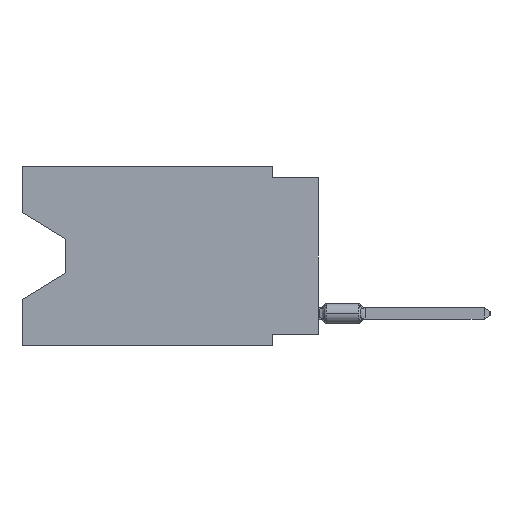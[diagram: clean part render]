
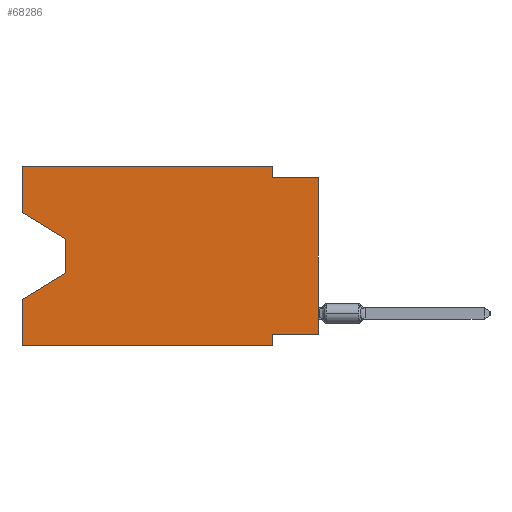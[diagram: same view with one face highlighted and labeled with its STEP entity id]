
A CAD part, left-side view. The second image highlights one B-rep face of the part: STEP entity #68286.
In plain terms, the highlighted planar face has unit normal (-1, 0, 0).
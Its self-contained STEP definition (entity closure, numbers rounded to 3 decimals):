
#536 = DIRECTION ( 'NONE',  ( 0., 0., -1. ) ) ;
#2184 = VECTOR ( 'NONE', #11105, 1000. ) ;
#2478 = EDGE_LOOP ( 'NONE', ( #61921, #39847, #47385, #11487, #75316, #33897, #19832, #38276, #31860, #69973, #53707, #51297 ) ) ;
#2851 = CARTESIAN_POINT ( 'NONE',  ( 0., 13.97, -4.013 ) ) ;
#3075 = EDGE_CURVE ( 'NONE', #68480, #20367, #23605, .T. ) ;
#3220 = VECTOR ( 'NONE', #50101, 1000. ) ;
#3346 = CARTESIAN_POINT ( 'NONE',  ( 0., 16.383, -9.906 ) ) ;
#4246 = DIRECTION ( 'NONE',  ( 0., -0.855, -0.519 ) ) ;
#6321 = CARTESIAN_POINT ( 'NONE',  ( 0., 16.383, 0. ) ) ;
#6379 = VECTOR ( 'NONE', #55084, 1000. ) ;
#6988 = EDGE_CURVE ( 'NONE', #44244, #68480, #17265, .T. ) ;
#7427 = VERTEX_POINT ( 'NONE', #64500 ) ;
#8883 = VERTEX_POINT ( 'NONE', #2851 ) ;
#10782 = CARTESIAN_POINT ( 'NONE',  ( 0., 2.54, -9.271 ) ) ;
#11105 = DIRECTION ( 'NONE',  ( 0., 1., 0. ) ) ;
#11487 = ORIENTED_EDGE ( 'NONE', *, *, #60969, .F. ) ;
#12878 = CARTESIAN_POINT ( 'NONE',  ( 0., 13.97, -4.013 ) ) ;
#13139 = LINE ( 'NONE', #38212, #6379 ) ;
#14327 = VERTEX_POINT ( 'NONE', #59065 ) ;
#14853 = LINE ( 'NONE', #53460, #24360 ) ;
#17265 = LINE ( 'NONE', #54662, #2184 ) ;
#17700 = EDGE_CURVE ( 'NONE', #64147, #47741, #14853, .T. ) ;
#17782 = CARTESIAN_POINT ( 'NONE',  ( 0., 16.383, -7.36 ) ) ;
#19370 = AXIS2_PLACEMENT_3D ( 'NONE', #6321, #31409, #25217 ) ;
#19832 = ORIENTED_EDGE ( 'NONE', *, *, #6988, .F. ) ;
#20367 = VERTEX_POINT ( 'NONE', #27792 ) ;
#20667 = DIRECTION ( 'NONE',  ( 0., 0., 1. ) ) ;
#22752 = DIRECTION ( 'NONE',  ( 0., -1., 0. ) ) ;
#23605 = LINE ( 'NONE', #79504, #75189 ) ;
#24106 = VERTEX_POINT ( 'NONE', #53067 ) ;
#24360 = VECTOR ( 'NONE', #71164, 1000. ) ;
#24638 = CARTESIAN_POINT ( 'NONE',  ( 0., 13.97, -5.893 ) ) ;
#25217 = DIRECTION ( 'NONE',  ( 0., 0., -1. ) ) ;
#26375 = CARTESIAN_POINT ( 'NONE',  ( 0., 0., 0. ) ) ;
#27792 = CARTESIAN_POINT ( 'NONE',  ( 0., 2.54, -9.906 ) ) ;
#28436 = CARTESIAN_POINT ( 'NONE',  ( 0., 0., -9.271 ) ) ;
#28966 = DIRECTION ( 'NONE',  ( 0., 0., -1. ) ) ;
#29402 = VECTOR ( 'NONE', #64873, 1000. ) ;
#30150 = LINE ( 'NONE', #49013, #41145 ) ;
#31319 = VERTEX_POINT ( 'NONE', #3346 ) ;
#31409 = DIRECTION ( 'NONE',  ( 1., 0., 0. ) ) ;
#31860 = ORIENTED_EDGE ( 'NONE', *, *, #35707, .F. ) ;
#33462 = EDGE_CURVE ( 'NONE', #8883, #46374, #49871, .T. ) ;
#33897 = ORIENTED_EDGE ( 'NONE', *, *, #3075, .F. ) ;
#34282 = LINE ( 'NONE', #35901, #72743 ) ;
#35707 = EDGE_CURVE ( 'NONE', #7427, #14327, #34282, .T. ) ;
#35901 = CARTESIAN_POINT ( 'NONE',  ( 0., 0., -0.635 ) ) ;
#36644 = CARTESIAN_POINT ( 'NONE',  ( 0., 16.383, 0. ) ) ;
#38212 = CARTESIAN_POINT ( 'NONE',  ( 0., 16.383, -9.906 ) ) ;
#38276 = ORIENTED_EDGE ( 'NONE', *, *, #45094, .T. ) ;
#38461 = EDGE_CURVE ( 'NONE', #46374, #81164, #68209, .T. ) ;
#38711 = DIRECTION ( 'NONE',  ( 0., 0., 1. ) ) ;
#39172 = LINE ( 'NONE', #76551, #41976 ) ;
#39847 = ORIENTED_EDGE ( 'NONE', *, *, #33462, .T. ) ;
#41145 = VECTOR ( 'NONE', #4246, 1000. ) ;
#41976 = VECTOR ( 'NONE', #20667, 1000. ) ;
#42107 = EDGE_CURVE ( 'NONE', #24106, #64147, #77945, .T. ) ;
#43710 = PLANE ( 'NONE',  #19370 ) ;
#44244 = VERTEX_POINT ( 'NONE', #28436 ) ;
#44283 = VECTOR ( 'NONE', #66007, 1000. ) ;
#45094 = EDGE_CURVE ( 'NONE', #44244, #14327, #57617, .T. ) ;
#45430 = EDGE_CURVE ( 'NONE', #31319, #20367, #13139, .T. ) ;
#46374 = VERTEX_POINT ( 'NONE', #62627 ) ;
#47385 = ORIENTED_EDGE ( 'NONE', *, *, #38461, .T. ) ;
#47741 = VERTEX_POINT ( 'NONE', #76685 ) ;
#49013 = CARTESIAN_POINT ( 'NONE',  ( 0., 16.383, -2.546 ) ) ;
#49871 = LINE ( 'NONE', #12878, #50375 ) ;
#50101 = DIRECTION ( 'NONE',  ( 0., 0.855, -0.519 ) ) ;
#50375 = VECTOR ( 'NONE', #536, 1000. ) ;
#50686 = FACE_OUTER_BOUND ( 'NONE', #2478, .T. ) ;
#51297 = ORIENTED_EDGE ( 'NONE', *, *, #42107, .F. ) ;
#53067 = CARTESIAN_POINT ( 'NONE',  ( 0., 16.383, -2.546 ) ) ;
#53276 = EDGE_CURVE ( 'NONE', #47741, #7427, #70635, .T. ) ;
#53460 = CARTESIAN_POINT ( 'NONE',  ( 0., 16.383, 0. ) ) ;
#53707 = ORIENTED_EDGE ( 'NONE', *, *, #17700, .F. ) ;
#54662 = CARTESIAN_POINT ( 'NONE',  ( 0., 0., -9.271 ) ) ;
#55084 = DIRECTION ( 'NONE',  ( 0., -1., 0. ) ) ;
#57617 = LINE ( 'NONE', #26375, #72050 ) ;
#59065 = CARTESIAN_POINT ( 'NONE',  ( 0., 0., -0.635 ) ) ;
#60969 = EDGE_CURVE ( 'NONE', #31319, #81164, #39172, .T. ) ;
#61921 = ORIENTED_EDGE ( 'NONE', *, *, #76586, .T. ) ;
#62627 = CARTESIAN_POINT ( 'NONE',  ( 0., 13.97, -5.893 ) ) ;
#64147 = VERTEX_POINT ( 'NONE', #36644 ) ;
#64500 = CARTESIAN_POINT ( 'NONE',  ( 0., 2.54, -0.635 ) ) ;
#64873 = DIRECTION ( 'NONE',  ( 0., 0., -1. ) ) ;
#66007 = DIRECTION ( 'NONE',  ( 0., 0., 1. ) ) ;
#68209 = LINE ( 'NONE', #24638, #3220 ) ;
#68286 = ADVANCED_FACE ( 'NONE', ( #50686 ), #43710, .F. ) ;
#68480 = VERTEX_POINT ( 'NONE', #10782 ) ;
#69973 = ORIENTED_EDGE ( 'NONE', *, *, #53276, .F. ) ;
#70635 = LINE ( 'NONE', #71042, #29402 ) ;
#71042 = CARTESIAN_POINT ( 'NONE',  ( 0., 2.54, 0. ) ) ;
#71164 = DIRECTION ( 'NONE',  ( 0., -1., 0. ) ) ;
#72050 = VECTOR ( 'NONE', #38711, 1000. ) ;
#72743 = VECTOR ( 'NONE', #22752, 1000. ) ;
#75189 = VECTOR ( 'NONE', #28966, 1000. ) ;
#75316 = ORIENTED_EDGE ( 'NONE', *, *, #45430, .T. ) ;
#76551 = CARTESIAN_POINT ( 'NONE',  ( 0., 16.383, 0. ) ) ;
#76586 = EDGE_CURVE ( 'NONE', #24106, #8883, #30150, .T. ) ;
#76685 = CARTESIAN_POINT ( 'NONE',  ( 0., 2.54, 0. ) ) ;
#77945 = LINE ( 'NONE', #78357, #44283 ) ;
#78357 = CARTESIAN_POINT ( 'NONE',  ( 0., 16.383, 0. ) ) ;
#79504 = CARTESIAN_POINT ( 'NONE',  ( 0., 2.54, -9.906 ) ) ;
#81164 = VERTEX_POINT ( 'NONE', #17782 ) ;
